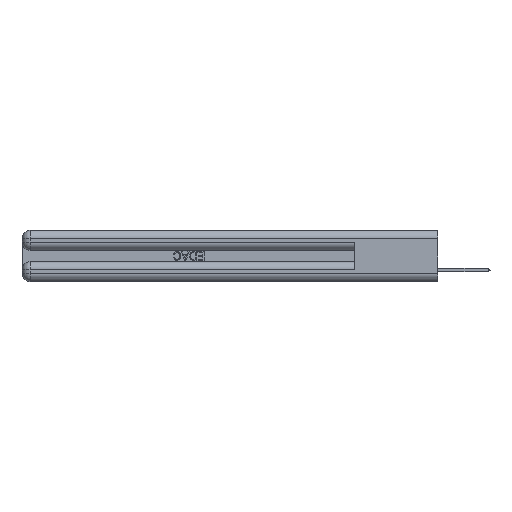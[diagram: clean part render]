
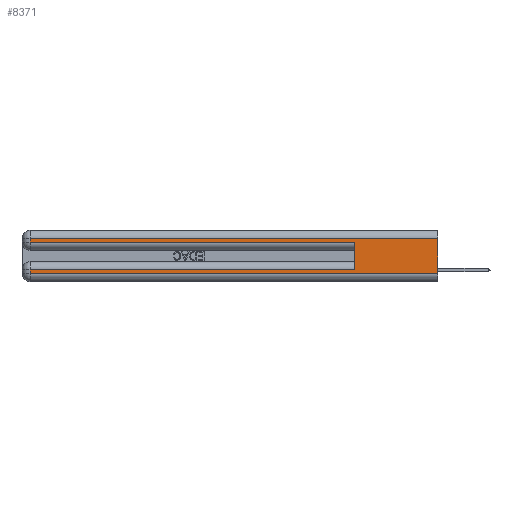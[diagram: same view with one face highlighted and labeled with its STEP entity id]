
A CAD part, left-side view. The second image highlights one B-rep face of the part: STEP entity #8371.
In plain terms, the highlighted planar face has unit normal (-1, 0, 0).
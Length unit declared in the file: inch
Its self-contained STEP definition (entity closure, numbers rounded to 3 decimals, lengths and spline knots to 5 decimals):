
#12 = LINE ( 'NONE', #14455, #26675 ) ;
#1854 = ORIENTED_EDGE ( 'NONE', *, *, #8179, .T. ) ;
#1926 = VERTEX_POINT ( 'NONE', #6343 ) ;
#2390 = VECTOR ( 'NONE', #6315, 39.37008 ) ;
#2407 = DIRECTION ( 'NONE',  ( 0., 1., 0. ) ) ;
#2784 = EDGE_CURVE ( 'NONE', #27006, #6880, #9654, .T. ) ;
#4566 = VERTEX_POINT ( 'NONE', #14004 ) ;
#5514 = VECTOR ( 'NONE', #36692, 39.37008 ) ;
#5608 = VERTEX_POINT ( 'NONE', #28895 ) ;
#6315 = DIRECTION ( 'NONE',  ( 0., -1., 0. ) ) ;
#6343 = CARTESIAN_POINT ( 'NONE',  ( 0., 0.6, 0.285 ) ) ;
#6880 = VERTEX_POINT ( 'NONE', #37304 ) ;
#7494 = ORIENTED_EDGE ( 'NONE', *, *, #11471, .T. ) ;
#7877 = ORIENTED_EDGE ( 'NONE', *, *, #23561, .T. ) ;
#8004 = DIRECTION ( 'NONE',  ( 0., 1., 0. ) ) ;
#8179 = EDGE_CURVE ( 'NONE', #10277, #27006, #11421, .T. ) ;
#8371 = ADVANCED_FACE ( 'NONE', ( #17396 ), #29050, .F. ) ;
#9073 = CARTESIAN_POINT ( 'NONE',  ( 0., 0., 0.31 ) ) ;
#9654 = LINE ( 'NONE', #23568, #15187 ) ;
#10027 = EDGE_CURVE ( 'NONE', #25196, #13880, #32030, .T. ) ;
#10277 = VERTEX_POINT ( 'NONE', #9073 ) ;
#11417 = CARTESIAN_POINT ( 'NONE',  ( 0., 0., 0.37 ) ) ;
#11421 = LINE ( 'NONE', #26206, #28932 ) ;
#11471 = EDGE_CURVE ( 'NONE', #13880, #4566, #17591, .T. ) ;
#13465 = AXIS2_PLACEMENT_3D ( 'NONE', #11417, #37835, #29182 ) ;
#13782 = EDGE_CURVE ( 'NONE', #10277, #4566, #33828, .T. ) ;
#13880 = VERTEX_POINT ( 'NONE', #25370 ) ;
#14004 = CARTESIAN_POINT ( 'NONE',  ( 0., 0., 0.06 ) ) ;
#14455 = CARTESIAN_POINT ( 'NONE',  ( 0., 0., 0.285 ) ) ;
#15173 = CARTESIAN_POINT ( 'NONE',  ( 0., 0., 0.06 ) ) ;
#15187 = VECTOR ( 'NONE', #34997, 39.37008 ) ;
#15817 = DIRECTION ( 'NONE',  ( 0., 0., -1. ) ) ;
#16837 = EDGE_CURVE ( 'NONE', #5608, #1926, #22530, .T. ) ;
#16859 = VECTOR ( 'NONE', #15817, 39.37008 ) ;
#17036 = CARTESIAN_POINT ( 'NONE',  ( 0., 2.94, 0.31 ) ) ;
#17113 = VECTOR ( 'NONE', #8004, 39.37008 ) ;
#17396 = FACE_OUTER_BOUND ( 'NONE', #26252, .T. ) ;
#17575 = ORIENTED_EDGE ( 'NONE', *, *, #29821, .T. ) ;
#17591 = LINE ( 'NONE', #15173, #2390 ) ;
#19310 = ORIENTED_EDGE ( 'NONE', *, *, #2784, .T. ) ;
#19859 = LINE ( 'NONE', #25888, #17113 ) ;
#20375 = ORIENTED_EDGE ( 'NONE', *, *, #10027, .T. ) ;
#22530 = LINE ( 'NONE', #33644, #5514 ) ;
#22645 = ORIENTED_EDGE ( 'NONE', *, *, #13782, .F. ) ;
#23541 = DIRECTION ( 'NONE',  ( 0., -1., 0. ) ) ;
#23561 = EDGE_CURVE ( 'NONE', #5608, #25196, #19859, .T. ) ;
#23568 = CARTESIAN_POINT ( 'NONE',  ( 0., 2.94, 0.37 ) ) ;
#24973 = ORIENTED_EDGE ( 'NONE', *, *, #16837, .F. ) ;
#25196 = VERTEX_POINT ( 'NONE', #30221 ) ;
#25370 = CARTESIAN_POINT ( 'NONE',  ( 0., 2.94, 0.06 ) ) ;
#25888 = CARTESIAN_POINT ( 'NONE',  ( 0., 0., 0.085 ) ) ;
#26206 = CARTESIAN_POINT ( 'NONE',  ( 0., 0., 0.31 ) ) ;
#26252 = EDGE_LOOP ( 'NONE', ( #22645, #1854, #19310, #17575, #24973, #7877, #20375, #7494 ) ) ;
#26675 = VECTOR ( 'NONE', #23541, 39.37008 ) ;
#27006 = VERTEX_POINT ( 'NONE', #17036 ) ;
#27513 = CARTESIAN_POINT ( 'NONE',  ( 0., 2.94, 0.37 ) ) ;
#28895 = CARTESIAN_POINT ( 'NONE',  ( 0., 0.6, 0.085 ) ) ;
#28932 = VECTOR ( 'NONE', #2407, 39.37008 ) ;
#29050 = PLANE ( 'NONE',  #13465 ) ;
#29182 = DIRECTION ( 'NONE',  ( 0., 0., -1. ) ) ;
#29821 = EDGE_CURVE ( 'NONE', #6880, #1926, #12, .T. ) ;
#30221 = CARTESIAN_POINT ( 'NONE',  ( 0., 2.94, 0.085 ) ) ;
#31070 = VECTOR ( 'NONE', #31148, 39.37008 ) ;
#31148 = DIRECTION ( 'NONE',  ( 0., 0., -1. ) ) ;
#32030 = LINE ( 'NONE', #27513, #16859 ) ;
#33644 = CARTESIAN_POINT ( 'NONE',  ( 0., 0.6, 0.145 ) ) ;
#33733 = CARTESIAN_POINT ( 'NONE',  ( 0., 0., 0.37 ) ) ;
#33828 = LINE ( 'NONE', #33733, #31070 ) ;
#34997 = DIRECTION ( 'NONE',  ( 0., 0., -1. ) ) ;
#36692 = DIRECTION ( 'NONE',  ( 0., 0., 1. ) ) ;
#37304 = CARTESIAN_POINT ( 'NONE',  ( 0., 2.94, 0.285 ) ) ;
#37835 = DIRECTION ( 'NONE',  ( 1., 0., 0. ) ) ;
